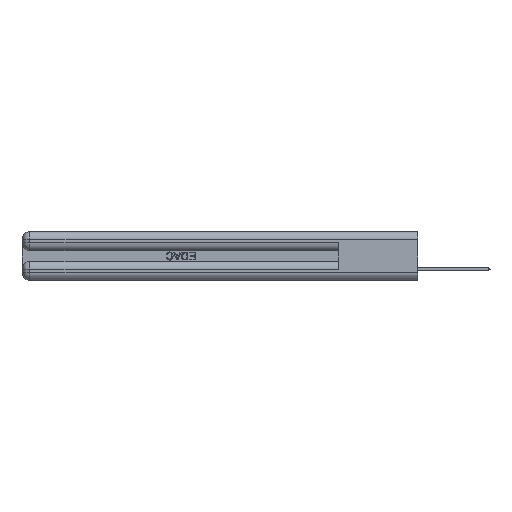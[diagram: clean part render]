
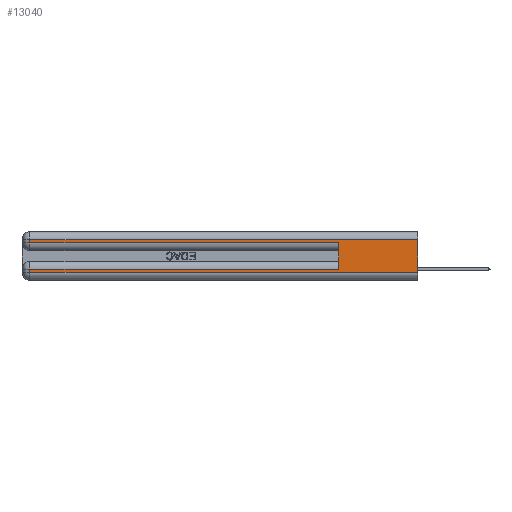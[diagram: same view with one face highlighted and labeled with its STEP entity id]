
A CAD part, left-side view. The second image highlights one B-rep face of the part: STEP entity #13040.
In plain terms, the highlighted planar face has unit normal (-1, 0, 0).
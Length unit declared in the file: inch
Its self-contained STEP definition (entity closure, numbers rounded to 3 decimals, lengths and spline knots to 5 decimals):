
#1156 = CARTESIAN_POINT ( 'NONE',  ( 0., 2.94, 0.285 ) ) ;
#1337 = EDGE_CURVE ( 'NONE', #3402, #36947, #24642, .T. ) ;
#1381 = CARTESIAN_POINT ( 'NONE',  ( 0., 0., 0.06 ) ) ;
#1413 = LINE ( 'NONE', #36887, #10354 ) ;
#1548 = DIRECTION ( 'NONE',  ( 0., 0., -1. ) ) ;
#2826 = ORIENTED_EDGE ( 'NONE', *, *, #1337, .T. ) ;
#3402 = VERTEX_POINT ( 'NONE', #3976 ) ;
#3569 = CARTESIAN_POINT ( 'NONE',  ( 0., 0.6, 0.085 ) ) ;
#3976 = CARTESIAN_POINT ( 'NONE',  ( 0., 2.94, 0.31 ) ) ;
#4132 = CARTESIAN_POINT ( 'NONE',  ( 0., 2.94, 0.37 ) ) ;
#4711 = CARTESIAN_POINT ( 'NONE',  ( 0., 0.6, 0.145 ) ) ;
#5000 = VECTOR ( 'NONE', #44219, 39.37008 ) ;
#5522 = EDGE_CURVE ( 'NONE', #36947, #41517, #21385, .T. ) ;
#5546 = CARTESIAN_POINT ( 'NONE',  ( 0., 0., 0.285 ) ) ;
#5576 = DIRECTION ( 'NONE',  ( 0., 1., 0. ) ) ;
#5703 = DIRECTION ( 'NONE',  ( 1., 0., 0. ) ) ;
#5759 = CARTESIAN_POINT ( 'NONE',  ( 0., 0.6, 0.285 ) ) ;
#6183 = LINE ( 'NONE', #4711, #5000 ) ;
#7817 = DIRECTION ( 'NONE',  ( 0., 1., 0. ) ) ;
#7951 = VECTOR ( 'NONE', #16414, 39.37008 ) ;
#8782 = DIRECTION ( 'NONE',  ( 0., 0., -1. ) ) ;
#9313 = LINE ( 'NONE', #31752, #21088 ) ;
#10354 = VECTOR ( 'NONE', #5576, 39.37008 ) ;
#11903 = EDGE_CURVE ( 'NONE', #30187, #13656, #36409, .T. ) ;
#12832 = DIRECTION ( 'NONE',  ( 0., -1., 0. ) ) ;
#13040 = ADVANCED_FACE ( 'NONE', ( #45320 ), #44736, .F. ) ;
#13210 = EDGE_CURVE ( 'NONE', #32409, #26574, #37413, .T. ) ;
#13566 = DIRECTION ( 'NONE',  ( 0., -1., 0. ) ) ;
#13656 = VERTEX_POINT ( 'NONE', #1381 ) ;
#15378 = ORIENTED_EDGE ( 'NONE', *, *, #22714, .T. ) ;
#15727 = CARTESIAN_POINT ( 'NONE',  ( 0., 0., 0.37 ) ) ;
#16414 = DIRECTION ( 'NONE',  ( 0., 0., -1. ) ) ;
#16707 = EDGE_LOOP ( 'NONE', ( #28852, #15378, #2826, #18034, #18052, #29438, #26524, #28464 ) ) ;
#17840 = CARTESIAN_POINT ( 'NONE',  ( 0., 0., 0.31 ) ) ;
#18034 = ORIENTED_EDGE ( 'NONE', *, *, #5522, .T. ) ;
#18052 = ORIENTED_EDGE ( 'NONE', *, *, #26623, .F. ) ;
#20795 = EDGE_CURVE ( 'NONE', #26574, #13656, #41258, .T. ) ;
#21088 = VECTOR ( 'NONE', #7817, 39.37008 ) ;
#21332 = VECTOR ( 'NONE', #40142, 39.37008 ) ;
#21385 = LINE ( 'NONE', #5546, #44718 ) ;
#22714 = EDGE_CURVE ( 'NONE', #30187, #3402, #1413, .T. ) ;
#24642 = LINE ( 'NONE', #4132, #21332 ) ;
#24836 = VECTOR ( 'NONE', #1548, 39.37008 ) ;
#26524 = ORIENTED_EDGE ( 'NONE', *, *, #13210, .T. ) ;
#26574 = VERTEX_POINT ( 'NONE', #32306 ) ;
#26623 = EDGE_CURVE ( 'NONE', #41881, #41517, #6183, .T. ) ;
#28464 = ORIENTED_EDGE ( 'NONE', *, *, #20795, .T. ) ;
#28852 = ORIENTED_EDGE ( 'NONE', *, *, #11903, .F. ) ;
#29438 = ORIENTED_EDGE ( 'NONE', *, *, #40063, .T. ) ;
#30187 = VERTEX_POINT ( 'NONE', #17840 ) ;
#31752 = CARTESIAN_POINT ( 'NONE',  ( 0., 0., 0.085 ) ) ;
#32306 = CARTESIAN_POINT ( 'NONE',  ( 0., 2.94, 0.06 ) ) ;
#32409 = VERTEX_POINT ( 'NONE', #42162 ) ;
#33288 = CARTESIAN_POINT ( 'NONE',  ( 0., 0., 0.37 ) ) ;
#34037 = VECTOR ( 'NONE', #13566, 39.37008 ) ;
#36409 = LINE ( 'NONE', #33288, #24836 ) ;
#36887 = CARTESIAN_POINT ( 'NONE',  ( 0., 0., 0.31 ) ) ;
#36947 = VERTEX_POINT ( 'NONE', #1156 ) ;
#37413 = LINE ( 'NONE', #41745, #7951 ) ;
#38891 = CARTESIAN_POINT ( 'NONE',  ( 0., 0., 0.06 ) ) ;
#40063 = EDGE_CURVE ( 'NONE', #41881, #32409, #9313, .T. ) ;
#40142 = DIRECTION ( 'NONE',  ( 0., 0., -1. ) ) ;
#41258 = LINE ( 'NONE', #38891, #34037 ) ;
#41517 = VERTEX_POINT ( 'NONE', #5759 ) ;
#41745 = CARTESIAN_POINT ( 'NONE',  ( 0., 2.94, 0.37 ) ) ;
#41881 = VERTEX_POINT ( 'NONE', #3569 ) ;
#42162 = CARTESIAN_POINT ( 'NONE',  ( 0., 2.94, 0.085 ) ) ;
#42797 = AXIS2_PLACEMENT_3D ( 'NONE', #15727, #5703, #8782 ) ;
#44219 = DIRECTION ( 'NONE',  ( 0., 0., 1. ) ) ;
#44718 = VECTOR ( 'NONE', #12832, 39.37008 ) ;
#44736 = PLANE ( 'NONE',  #42797 ) ;
#45320 = FACE_OUTER_BOUND ( 'NONE', #16707, .T. ) ;
